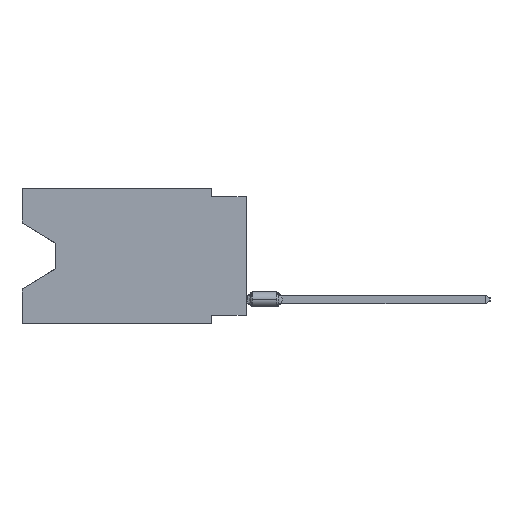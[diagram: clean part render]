
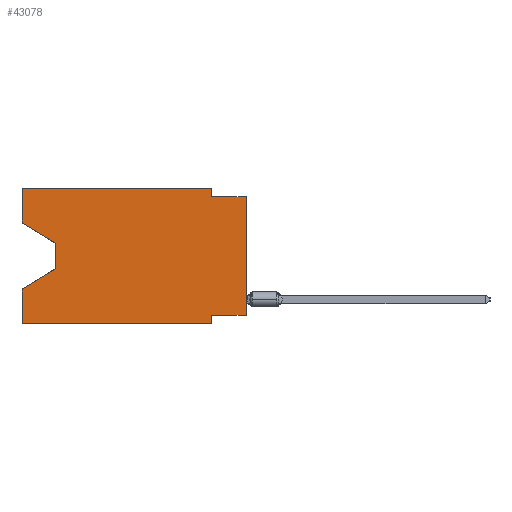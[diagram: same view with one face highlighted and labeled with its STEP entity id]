
A CAD part, left-side view. The second image highlights one B-rep face of the part: STEP entity #43078.
In plain terms, the highlighted planar face has unit normal (-1, 0, 0).
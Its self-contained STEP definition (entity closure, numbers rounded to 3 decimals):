
#267 = CARTESIAN_POINT ( 'NONE',  ( 0., 0., -0.635 ) ) ;
#797 = VECTOR ( 'NONE', #36605, 1000. ) ;
#1160 = ORIENTED_EDGE ( 'NONE', *, *, #14851, .F. ) ;
#1255 = VECTOR ( 'NONE', #10914, 1000. ) ;
#1610 = VERTEX_POINT ( 'NONE', #25170 ) ;
#2789 = ORIENTED_EDGE ( 'NONE', *, *, #36106, .F. ) ;
#3762 = CARTESIAN_POINT ( 'NONE',  ( 0., 16.383, -7.36 ) ) ;
#3998 = LINE ( 'NONE', #33049, #34199 ) ;
#4046 = VERTEX_POINT ( 'NONE', #3762 ) ;
#4299 = DIRECTION ( 'NONE',  ( 1., 0., 0. ) ) ;
#4660 = EDGE_CURVE ( 'NONE', #42167, #39689, #33530, .T. ) ;
#5236 = DIRECTION ( 'NONE',  ( 0., 0., -1. ) ) ;
#5430 = CARTESIAN_POINT ( 'NONE',  ( 0., 13.97, -4.013 ) ) ;
#5618 = LINE ( 'NONE', #46064, #32742 ) ;
#6859 = LINE ( 'NONE', #18053, #44824 ) ;
#7119 = LINE ( 'NONE', #43310, #47050 ) ;
#8142 = CARTESIAN_POINT ( 'NONE',  ( 0., 0., 0. ) ) ;
#8989 = LINE ( 'NONE', #5430, #41603 ) ;
#10385 = VECTOR ( 'NONE', #37196, 1000. ) ;
#10914 = DIRECTION ( 'NONE',  ( 0., -0.855, -0.519 ) ) ;
#11729 = LINE ( 'NONE', #8142, #10385 ) ;
#13846 = CARTESIAN_POINT ( 'NONE',  ( 0., 0., -0.635 ) ) ;
#14325 = ORIENTED_EDGE ( 'NONE', *, *, #44826, .T. ) ;
#14509 = VECTOR ( 'NONE', #44594, 1000. ) ;
#14851 = EDGE_CURVE ( 'NONE', #31816, #36151, #26132, .T. ) ;
#15154 = DIRECTION ( 'NONE',  ( 0., -1., 0. ) ) ;
#15174 = EDGE_CURVE ( 'NONE', #1610, #45992, #5618, .T. ) ;
#16196 = VECTOR ( 'NONE', #43737, 1000. ) ;
#16295 = ORIENTED_EDGE ( 'NONE', *, *, #35941, .F. ) ;
#16911 = CARTESIAN_POINT ( 'NONE',  ( 0., 16.383, -2.546 ) ) ;
#17548 = CARTESIAN_POINT ( 'NONE',  ( 0., 13.97, -4.013 ) ) ;
#18053 = CARTESIAN_POINT ( 'NONE',  ( 0., 2.54, 0. ) ) ;
#18478 = CARTESIAN_POINT ( 'NONE',  ( 0., 2.54, -9.906 ) ) ;
#18721 = LINE ( 'NONE', #26101, #37208 ) ;
#19095 = CARTESIAN_POINT ( 'NONE',  ( 0., 16.383, -9.906 ) ) ;
#19147 = CARTESIAN_POINT ( 'NONE',  ( 0., 13.97, -5.893 ) ) ;
#19775 = AXIS2_PLACEMENT_3D ( 'NONE', #41418, #4299, #5236 ) ;
#19956 = VERTEX_POINT ( 'NONE', #38607 ) ;
#20242 = VERTEX_POINT ( 'NONE', #267 ) ;
#21021 = EDGE_CURVE ( 'NONE', #39162, #4046, #26510, .T. ) ;
#21256 = VECTOR ( 'NONE', #33666, 1000. ) ;
#22083 = CARTESIAN_POINT ( 'NONE',  ( 0., 0., -9.271 ) ) ;
#22676 = CARTESIAN_POINT ( 'NONE',  ( 0., 13.97, -5.893 ) ) ;
#22913 = ORIENTED_EDGE ( 'NONE', *, *, #26550, .F. ) ;
#23268 = CARTESIAN_POINT ( 'NONE',  ( 0., 2.54, -9.271 ) ) ;
#23744 = DIRECTION ( 'NONE',  ( 0., 0., -1. ) ) ;
#24392 = ORIENTED_EDGE ( 'NONE', *, *, #21021, .T. ) ;
#25170 = CARTESIAN_POINT ( 'NONE',  ( 0., 16.383, 0. ) ) ;
#25469 = ORIENTED_EDGE ( 'NONE', *, *, #37632, .T. ) ;
#26101 = CARTESIAN_POINT ( 'NONE',  ( 0., 16.383, -9.906 ) ) ;
#26132 = LINE ( 'NONE', #22083, #797 ) ;
#26445 = FACE_OUTER_BOUND ( 'NONE', #31643, .T. ) ;
#26510 = LINE ( 'NONE', #19147, #21256 ) ;
#26550 = EDGE_CURVE ( 'NONE', #44324, #4046, #7119, .T. ) ;
#26877 = CARTESIAN_POINT ( 'NONE',  ( 0., 2.54, 0. ) ) ;
#27196 = CARTESIAN_POINT ( 'NONE',  ( 0., 16.383, 0. ) ) ;
#27213 = ORIENTED_EDGE ( 'NONE', *, *, #15174, .F. ) ;
#28887 = EDGE_CURVE ( 'NONE', #19956, #20242, #42625, .T. ) ;
#30489 = PLANE ( 'NONE',  #19775 ) ;
#31435 = ORIENTED_EDGE ( 'NONE', *, *, #33043, .T. ) ;
#31643 = EDGE_LOOP ( 'NONE', ( #42542, #14325, #24392, #22913, #25469, #2789, #1160, #31435, #44359, #16295, #27213, #36537 ) ) ;
#31816 = VERTEX_POINT ( 'NONE', #33095 ) ;
#32568 = DIRECTION ( 'NONE',  ( 0., 0., -1. ) ) ;
#32742 = VECTOR ( 'NONE', #39166, 1000. ) ;
#33043 = EDGE_CURVE ( 'NONE', #31816, #20242, #11729, .T. ) ;
#33049 = CARTESIAN_POINT ( 'NONE',  ( 0., 2.54, -9.906 ) ) ;
#33095 = CARTESIAN_POINT ( 'NONE',  ( 0., 0., -9.271 ) ) ;
#33281 = CARTESIAN_POINT ( 'NONE',  ( 0., 16.383, -2.546 ) ) ;
#33530 = LINE ( 'NONE', #33281, #1255 ) ;
#33666 = DIRECTION ( 'NONE',  ( 0., 0.855, -0.519 ) ) ;
#34199 = VECTOR ( 'NONE', #23744, 1000. ) ;
#34483 = DIRECTION ( 'NONE',  ( 0., 0., -1. ) ) ;
#35941 = EDGE_CURVE ( 'NONE', #45992, #19956, #6859, .T. ) ;
#36106 = EDGE_CURVE ( 'NONE', #36151, #39046, #3998, .T. ) ;
#36151 = VERTEX_POINT ( 'NONE', #23268 ) ;
#36537 = ORIENTED_EDGE ( 'NONE', *, *, #43849, .F. ) ;
#36605 = DIRECTION ( 'NONE',  ( 0., 1., 0. ) ) ;
#37196 = DIRECTION ( 'NONE',  ( 0., 0., 1. ) ) ;
#37208 = VECTOR ( 'NONE', #15154, 1000. ) ;
#37632 = EDGE_CURVE ( 'NONE', #44324, #39046, #18721, .T. ) ;
#38607 = CARTESIAN_POINT ( 'NONE',  ( 0., 2.54, -0.635 ) ) ;
#39046 = VERTEX_POINT ( 'NONE', #18478 ) ;
#39162 = VERTEX_POINT ( 'NONE', #22676 ) ;
#39166 = DIRECTION ( 'NONE',  ( 0., -1., 0. ) ) ;
#39689 = VERTEX_POINT ( 'NONE', #17548 ) ;
#41418 = CARTESIAN_POINT ( 'NONE',  ( 0., 16.383, 0. ) ) ;
#41603 = VECTOR ( 'NONE', #34483, 1000. ) ;
#41707 = LINE ( 'NONE', #27196, #14509 ) ;
#42167 = VERTEX_POINT ( 'NONE', #16911 ) ;
#42542 = ORIENTED_EDGE ( 'NONE', *, *, #4660, .T. ) ;
#42607 = DIRECTION ( 'NONE',  ( 0., 0., 1. ) ) ;
#42625 = LINE ( 'NONE', #13846, #16196 ) ;
#43078 = ADVANCED_FACE ( 'NONE', ( #26445 ), #30489, .F. ) ;
#43310 = CARTESIAN_POINT ( 'NONE',  ( 0., 16.383, 0. ) ) ;
#43737 = DIRECTION ( 'NONE',  ( 0., -1., 0. ) ) ;
#43849 = EDGE_CURVE ( 'NONE', #42167, #1610, #41707, .T. ) ;
#44324 = VERTEX_POINT ( 'NONE', #19095 ) ;
#44359 = ORIENTED_EDGE ( 'NONE', *, *, #28887, .F. ) ;
#44594 = DIRECTION ( 'NONE',  ( 0., 0., 1. ) ) ;
#44824 = VECTOR ( 'NONE', #32568, 1000. ) ;
#44826 = EDGE_CURVE ( 'NONE', #39689, #39162, #8989, .T. ) ;
#45992 = VERTEX_POINT ( 'NONE', #26877 ) ;
#46064 = CARTESIAN_POINT ( 'NONE',  ( 0., 16.383, 0. ) ) ;
#47050 = VECTOR ( 'NONE', #42607, 1000. ) ;
